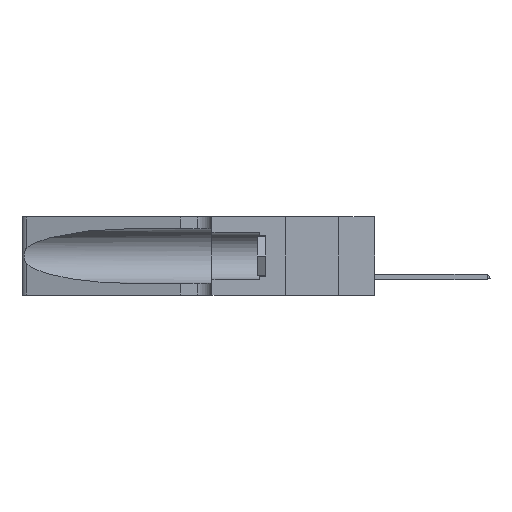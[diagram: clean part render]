
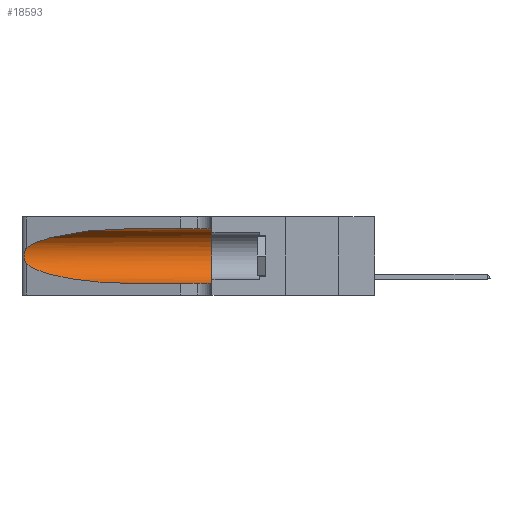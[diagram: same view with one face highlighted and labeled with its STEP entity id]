
A CAD part, left-side view. The second image highlights one B-rep face of the part: STEP entity #18593.
In plain terms, the highlighted cylindrical face has radius 3.308 mm (diameter 6.617 mm), a partial arc.
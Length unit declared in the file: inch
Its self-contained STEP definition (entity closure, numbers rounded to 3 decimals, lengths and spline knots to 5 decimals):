
#23 = ORIENTED_EDGE ( 'NONE', *, *, #3900, .T. ) ;
#904 = VERTEX_POINT ( 'NONE', #8767 ) ;
#1122 = EDGE_CURVE ( 'NONE', #2641, #15123, #18966, .T. ) ;
#1130 = LINE ( 'NONE', #19964, #22077 ) ;
#1339 = VECTOR ( 'NONE', #11746, 39.37008 ) ;
#1631 = VERTEX_POINT ( 'NONE', #5311 ) ;
#1650 = CARTESIAN_POINT ( 'NONE',  ( 0.18966, 0.96281, 0.05475 ) ) ;
#2077 = EDGE_LOOP ( 'NONE', ( #23, #18181, #8714, #22564, #19746, #9595 ) ) ;
#2641 = VERTEX_POINT ( 'NONE', #6660 ) ;
#3099 = CARTESIAN_POINT ( 'NONE',  ( 0.1305, 1.61858, 0.31525 ) ) ;
#3225 = CARTESIAN_POINT ( 'NONE',  ( 0.25639, 1.23186, 0.15144 ) ) ;
#3900 = EDGE_CURVE ( 'NONE', #904, #2641, #21088, .T. ) ;
#4135 = CARTESIAN_POINT ( 'NONE',  ( 0.25487, 1.22718, 0.14631 ) ) ;
#5067 = CARTESIAN_POINT ( 'NONE',  ( 0.1305, 1.61858, 0.185 ) ) ;
#5161 = CARTESIAN_POINT ( 'NONE',  ( 0.25487, 1.22718, 0.22369 ) ) ;
#5183 = CARTESIAN_POINT ( 'NONE',  ( 0.1305, 0.72297, 0.05475 ) ) ;
#5311 = CARTESIAN_POINT ( 'NONE',  ( 0.1305, 0.72297, 0.05475 ) ) ;
#5322 = CARTESIAN_POINT ( 'NONE',  ( 0.2373, 1.15595, 0.28018 ) ) ;
#5328 = CARTESIAN_POINT ( 'NONE',  ( 0.25639, 1.23184, 0.21858 ) ) ;
#5413 = VERTEX_POINT ( 'NONE', #14435 ) ;
#5933 = VERTEX_POINT ( 'NONE', #14383 ) ;
#6564 = LINE ( 'NONE', #3099, #1339 ) ;
#6660 = CARTESIAN_POINT ( 'NONE',  ( 0.25487, 1.22718, 0.22369 ) ) ;
#6706 = CARTESIAN_POINT ( 'NONE',  ( 0.25787, 1.23484, 0.2124 ) ) ;
#6866 = CARTESIAN_POINT ( 'NONE',  ( 0.26018, 1.23835, 0.19895 ) ) ;
#6928 = DIRECTION ( 'NONE',  ( 0., 0., -1. ) ) ;
#7410 =( BOUNDED_CURVE ( )  B_SPLINE_CURVE ( 3, ( #10739, #21290, #1650, #5183 ),
 .UNSPECIFIED., .F., .F. ) 
 B_SPLINE_CURVE_WITH_KNOTS ( ( 4, 4 ),
 ( 3.44316, 4.71239 ),
 .UNSPECIFIED. ) 
 CURVE ( )  GEOMETRIC_REPRESENTATION_ITEM ( )  RATIONAL_B_SPLINE_CURVE ( ( 1., 0.87, 0.87, 1. ) ) 
 REPRESENTATION_ITEM ( '' )  );
#8486 = CARTESIAN_POINT ( 'NONE',  ( 0.25856, 1.23593, 0.16098 ) ) ;
#8714 = ORIENTED_EDGE ( 'NONE', *, *, #8997, .T. ) ;
#8718 = CARTESIAN_POINT ( 'NONE',  ( 0.1305, 0.72297, 0.31525 ) ) ;
#8767 = CARTESIAN_POINT ( 'NONE',  ( 0.1305, 0.72297, 0.31525 ) ) ;
#8997 = EDGE_CURVE ( 'NONE', #15123, #1631, #7410, .T. ) ;
#9595 = ORIENTED_EDGE ( 'NONE', *, *, #17591, .F. ) ;
#9719 = AXIS2_PLACEMENT_3D ( 'NONE', #19879, #12975, #21675 ) ;
#10345 = CARTESIAN_POINT ( 'NONE',  ( 0.26075, 1.23896, 0.19203 ) ) ;
#10739 = CARTESIAN_POINT ( 'NONE',  ( 0.25487, 1.22718, 0.14631 ) ) ;
#11746 = DIRECTION ( 'NONE',  ( 0., -1., 0. ) ) ;
#12169 = CARTESIAN_POINT ( 'NONE',  ( 0.25854, 1.2359, 0.20912 ) ) ;
#12975 = DIRECTION ( 'NONE',  ( 0., 1., 0. ) ) ;
#13801 = CARTESIAN_POINT ( 'NONE',  ( 0.26017, 1.23833, 0.17102 ) ) ;
#13936 = DIRECTION ( 'NONE',  ( 0., -1., 0. ) ) ;
#13958 = CARTESIAN_POINT ( 'NONE',  ( 0.25555, 1.22993, 0.14849 ) ) ;
#14383 = CARTESIAN_POINT ( 'NONE',  ( 0.1305, 0.35, 0.05475 ) ) ;
#14435 = CARTESIAN_POINT ( 'NONE',  ( 0.1305, 0.35, 0.31525 ) ) ;
#15123 = VERTEX_POINT ( 'NONE', #4135 ) ;
#15538 = AXIS2_PLACEMENT_3D ( 'NONE', #5067, #13936, #6928 ) ;
#15720 = FACE_OUTER_BOUND ( 'NONE', #2077, .T. ) ;
#15763 = CARTESIAN_POINT ( 'NONE',  ( 0.18966, 0.96281, 0.31525 ) ) ;
#16348 = DIRECTION ( 'NONE',  ( 0., -1., 0. ) ) ;
#17490 = CARTESIAN_POINT ( 'NONE',  ( 0.26075, 1.23896, 0.178 ) ) ;
#17591 = EDGE_CURVE ( 'NONE', #904, #5413, #6564, .T. ) ;
#18181 = ORIENTED_EDGE ( 'NONE', *, *, #1122, .T. ) ;
#18593 = ADVANCED_FACE ( 'NONE', ( #15720 ), #19054, .F. ) ;
#18966 = B_SPLINE_CURVE_WITH_KNOTS ( 'NONE', 3,
 ( #22707, #19029, #5328, #6706, #12169, #6866, #10345, #17490, #13801, #8486, #21025, #3225, #13958, #22572 ),
 .UNSPECIFIED., .F., .F.,
 ( 4, 2, 2, 2, 2, 2, 4 ),
 ( 0., 0.00027, 0.00053, 0.00107, 0.0016, 0.00187, 0.00214 ),
 .UNSPECIFIED. ) ;
#19029 = CARTESIAN_POINT ( 'NONE',  ( 0.25555, 1.22994, 0.2215 ) ) ;
#19054 = CYLINDRICAL_SURFACE ( 'NONE', #15538, 0.13025 ) ;
#19089 = EDGE_CURVE ( 'NONE', #5413, #5933, #19293, .T. ) ;
#19293 = CIRCLE ( 'NONE', #9719, 0.13025 ) ;
#19407 = EDGE_CURVE ( 'NONE', #1631, #5933, #1130, .T. ) ;
#19746 = ORIENTED_EDGE ( 'NONE', *, *, #19089, .F. ) ;
#19879 = CARTESIAN_POINT ( 'NONE',  ( 0.1305, 0.35, 0.185 ) ) ;
#19964 = CARTESIAN_POINT ( 'NONE',  ( 0.1305, 1.61858, 0.05475 ) ) ;
#21025 = CARTESIAN_POINT ( 'NONE',  ( 0.25789, 1.23486, 0.15765 ) ) ;
#21088 =( BOUNDED_CURVE ( )  B_SPLINE_CURVE ( 3, ( #8718, #15763, #5322, #5161 ),
 .UNSPECIFIED., .F., .F. ) 
 B_SPLINE_CURVE_WITH_KNOTS ( ( 4, 4 ),
 ( 1.5708, 2.84003 ),
 .UNSPECIFIED. ) 
 CURVE ( )  GEOMETRIC_REPRESENTATION_ITEM ( )  RATIONAL_B_SPLINE_CURVE ( ( 1., 0.87, 0.87, 1. ) ) 
 REPRESENTATION_ITEM ( '' )  );
#21290 = CARTESIAN_POINT ( 'NONE',  ( 0.2373, 1.15595, 0.08982 ) ) ;
#21675 = DIRECTION ( 'NONE',  ( 0., 0., 1. ) ) ;
#22077 = VECTOR ( 'NONE', #16348, 39.37008 ) ;
#22564 = ORIENTED_EDGE ( 'NONE', *, *, #19407, .T. ) ;
#22572 = CARTESIAN_POINT ( 'NONE',  ( 0.25487, 1.22718, 0.14631 ) ) ;
#22707 = CARTESIAN_POINT ( 'NONE',  ( 0.25487, 1.22718, 0.22369 ) ) ;
